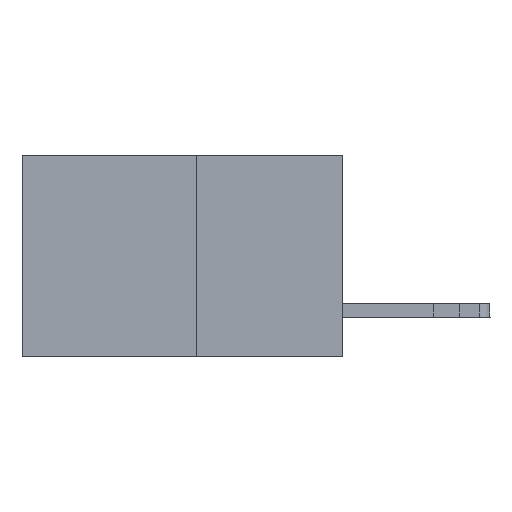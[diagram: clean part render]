
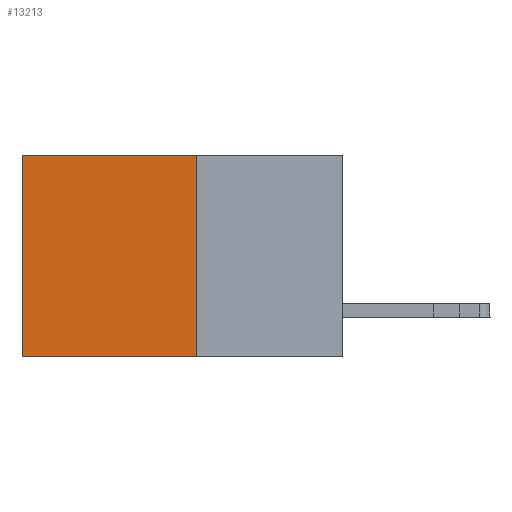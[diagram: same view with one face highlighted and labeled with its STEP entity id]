
A CAD part, left-side view. The second image highlights one B-rep face of the part: STEP entity #13213.
In plain terms, the highlighted planar face has unit normal (-1, 0, 0).
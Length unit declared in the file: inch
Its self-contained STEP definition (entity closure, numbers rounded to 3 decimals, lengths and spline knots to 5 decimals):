
#654 = CARTESIAN_POINT ( 'NONE',  ( 0.277, 0.59, -0.37 ) ) ;
#1806 = LINE ( 'NONE', #1893, #7032 ) ;
#1893 = CARTESIAN_POINT ( 'NONE',  ( 0.277, 0.59, -0.37 ) ) ;
#2678 = EDGE_CURVE ( 'NONE', #10126, #6550, #1806, .T. ) ;
#2716 = ORIENTED_EDGE ( 'NONE', *, *, #6813, .T. ) ;
#2789 = AXIS2_PLACEMENT_3D ( 'NONE', #11331, #10063, #14111 ) ;
#3644 = EDGE_CURVE ( 'NONE', #17360, #12917, #8584, .T. ) ;
#4410 = CARTESIAN_POINT ( 'NONE',  ( 0.277, 0.27, 0. ) ) ;
#5854 = PLANE ( 'NONE',  #2789 ) ;
#6274 = VECTOR ( 'NONE', #15422, 39.37008 ) ;
#6550 = VERTEX_POINT ( 'NONE', #654 ) ;
#6678 = CARTESIAN_POINT ( 'NONE',  ( 0.277, 0.27, -0.37 ) ) ;
#6813 = EDGE_CURVE ( 'NONE', #17360, #10126, #16736, .T. ) ;
#7032 = VECTOR ( 'NONE', #7279, 39.37008 ) ;
#7279 = DIRECTION ( 'NONE',  ( 0., 0., -1. ) ) ;
#7740 = ORIENTED_EDGE ( 'NONE', *, *, #2678, .T. ) ;
#8207 = LINE ( 'NONE', #6678, #10157 ) ;
#8584 = LINE ( 'NONE', #9932, #6274 ) ;
#9212 = EDGE_LOOP ( 'NONE', ( #7740, #14047, #17324, #2716 ) ) ;
#9932 = CARTESIAN_POINT ( 'NONE',  ( 0.277, 0.27, -0.37 ) ) ;
#10061 = DIRECTION ( 'NONE',  ( 0., 1., 0. ) ) ;
#10063 = DIRECTION ( 'NONE',  ( 1., 0., 0. ) ) ;
#10126 = VERTEX_POINT ( 'NONE', #17034 ) ;
#10157 = VECTOR ( 'NONE', #14862, 39.37008 ) ;
#11331 = CARTESIAN_POINT ( 'NONE',  ( 0.277, 0.27, -0.37 ) ) ;
#11500 = CARTESIAN_POINT ( 'NONE',  ( 0.277, 0.27, 0. ) ) ;
#12063 = CARTESIAN_POINT ( 'NONE',  ( 0.277, 0.27, -0.37 ) ) ;
#12917 = VERTEX_POINT ( 'NONE', #12063 ) ;
#13213 = ADVANCED_FACE ( 'NONE', ( #17002 ), #5854, .F. ) ;
#14047 = ORIENTED_EDGE ( 'NONE', *, *, #15558, .F. ) ;
#14105 = VECTOR ( 'NONE', #10061, 39.37008 ) ;
#14111 = DIRECTION ( 'NONE',  ( 0., 0., -1. ) ) ;
#14862 = DIRECTION ( 'NONE',  ( 0., 1., 0. ) ) ;
#15422 = DIRECTION ( 'NONE',  ( 0., 0., -1. ) ) ;
#15558 = EDGE_CURVE ( 'NONE', #12917, #6550, #8207, .T. ) ;
#16736 = LINE ( 'NONE', #11500, #14105 ) ;
#17002 = FACE_OUTER_BOUND ( 'NONE', #9212, .T. ) ;
#17034 = CARTESIAN_POINT ( 'NONE',  ( 0.277, 0.59, 0. ) ) ;
#17324 = ORIENTED_EDGE ( 'NONE', *, *, #3644, .F. ) ;
#17360 = VERTEX_POINT ( 'NONE', #4410 ) ;
